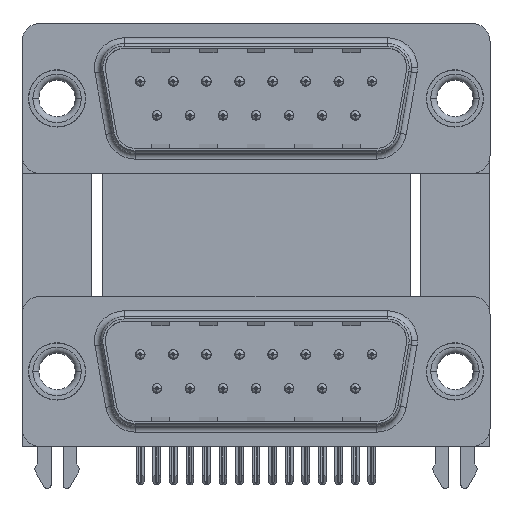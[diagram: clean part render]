
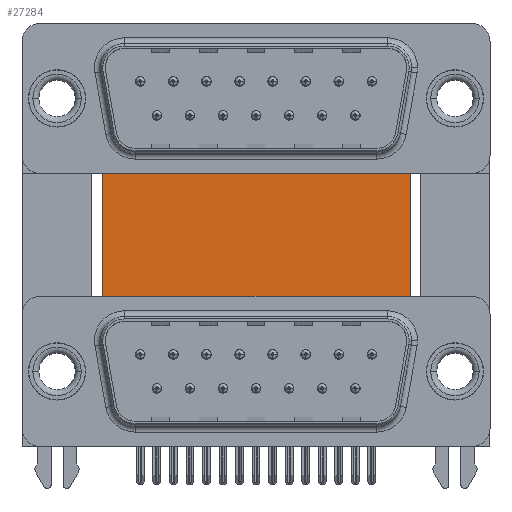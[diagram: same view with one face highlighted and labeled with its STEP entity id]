
A CAD part, top view. The second image highlights one B-rep face of the part: STEP entity #27284.
In plain terms, the highlighted planar face has unit normal (0, 0, 1).
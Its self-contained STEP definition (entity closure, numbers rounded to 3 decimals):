
#901 = DIRECTION ( 'NONE',  ( 0., 0., -1. ) ) ;
#3798 = ORIENTED_EDGE ( 'NONE', *, *, #29494, .T. ) ;
#4123 = VECTOR ( 'NONE', #5216, 1000. ) ;
#4427 = LINE ( 'NONE', #4567, #8185 ) ;
#4567 = CARTESIAN_POINT ( 'NONE',  ( 3.79, -3.735, -12. ) ) ;
#5216 = DIRECTION ( 'NONE',  ( 0., -1., 0. ) ) ;
#6475 = DIRECTION ( 'NONE',  ( 1., 0., 0. ) ) ;
#6618 = EDGE_CURVE ( 'NONE', #25881, #7257, #18969, .T. ) ;
#6881 = ORIENTED_EDGE ( 'NONE', *, *, #11614, .F. ) ;
#7257 = VERTEX_POINT ( 'NONE', #25080 ) ;
#7264 = CARTESIAN_POINT ( 'NONE',  ( 3.79, 16.585, -12. ) ) ;
#7353 = CARTESIAN_POINT ( 'NONE',  ( 3.79, 16.585, -12. ) ) ;
#7408 = CARTESIAN_POINT ( 'NONE',  ( 29.58, 16.585, -12. ) ) ;
#8185 = VECTOR ( 'NONE', #26235, 1000. ) ;
#8413 = PLANE ( 'NONE',  #16506 ) ;
#9159 = VERTEX_POINT ( 'NONE', #23796 ) ;
#9551 = ORIENTED_EDGE ( 'NONE', *, *, #18550, .T. ) ;
#10291 = VECTOR ( 'NONE', #6475, 1000. ) ;
#11614 = EDGE_CURVE ( 'NONE', #30666, #25881, #28695, .T. ) ;
#12759 = LINE ( 'NONE', #20246, #22479 ) ;
#16506 = AXIS2_PLACEMENT_3D ( 'NONE', #27419, #901, #22125 ) ;
#16852 = EDGE_LOOP ( 'NONE', ( #9551, #26058, #6881, #3798 ) ) ;
#17448 = DIRECTION ( 'NONE',  ( 0., -1., 0. ) ) ;
#18550 = EDGE_CURVE ( 'NONE', #9159, #7257, #4427, .T. ) ;
#18969 = LINE ( 'NONE', #7408, #4123 ) ;
#20246 = CARTESIAN_POINT ( 'NONE',  ( 3.79, 16.585, -12. ) ) ;
#21663 = CARTESIAN_POINT ( 'NONE',  ( 29.58, 16.585, -12. ) ) ;
#22125 = DIRECTION ( 'NONE',  ( -1., 0., 0. ) ) ;
#22479 = VECTOR ( 'NONE', #17448, 1000. ) ;
#23796 = CARTESIAN_POINT ( 'NONE',  ( 3.79, -3.735, -12. ) ) ;
#24617 = FACE_OUTER_BOUND ( 'NONE', #16852, .T. ) ;
#25080 = CARTESIAN_POINT ( 'NONE',  ( 29.58, -3.735, -12. ) ) ;
#25881 = VERTEX_POINT ( 'NONE', #21663 ) ;
#26058 = ORIENTED_EDGE ( 'NONE', *, *, #6618, .F. ) ;
#26235 = DIRECTION ( 'NONE',  ( 1., 0., 0. ) ) ;
#27284 = ADVANCED_FACE ( 'NONE', ( #24617 ), #8413, .F. ) ;
#27419 = CARTESIAN_POINT ( 'NONE',  ( 3.79, 16.585, -12. ) ) ;
#28695 = LINE ( 'NONE', #7353, #10291 ) ;
#29494 = EDGE_CURVE ( 'NONE', #30666, #9159, #12759, .T. ) ;
#30666 = VERTEX_POINT ( 'NONE', #7264 ) ;
